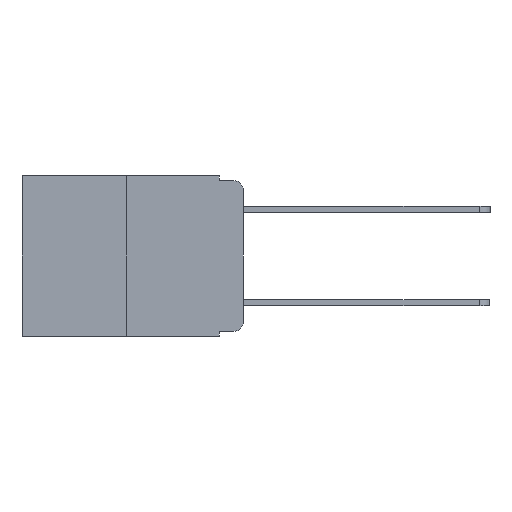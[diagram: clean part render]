
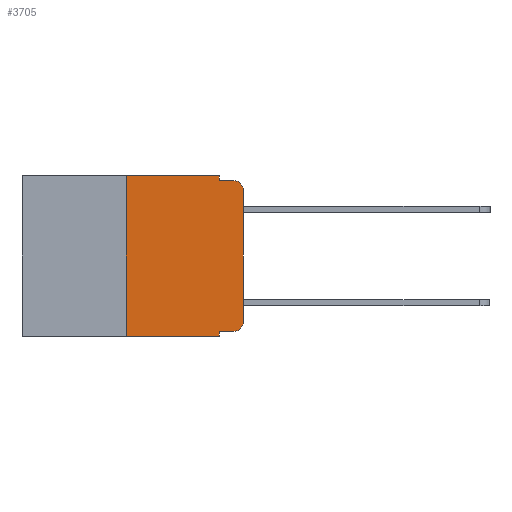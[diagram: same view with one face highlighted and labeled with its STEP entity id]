
A CAD part, left-side view. The second image highlights one B-rep face of the part: STEP entity #3705.
In plain terms, the highlighted planar face has unit normal (-1, 0, 0).
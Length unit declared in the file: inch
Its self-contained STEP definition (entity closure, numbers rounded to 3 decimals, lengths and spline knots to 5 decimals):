
#115 = DIRECTION ( 'NONE',  ( 0., 0., -1. ) ) ;
#124 = EDGE_CURVE ( 'NONE', #6362, #11952, #1915, .T. ) ;
#329 = DIRECTION ( 'NONE',  ( 0., 0., -1. ) ) ;
#531 = ORIENTED_EDGE ( 'NONE', *, *, #14129, .T. ) ;
#586 = CARTESIAN_POINT ( 'NONE',  ( 0., 0.25, -0.343 ) ) ;
#763 = ORIENTED_EDGE ( 'NONE', *, *, #14871, .F. ) ;
#785 = ORIENTED_EDGE ( 'NONE', *, *, #124, .F. ) ;
#868 = EDGE_CURVE ( 'NONE', #14524, #15082, #9923, .T. ) ;
#1090 = EDGE_CURVE ( 'NONE', #14524, #1942, #3526, .T. ) ;
#1223 = ORIENTED_EDGE ( 'NONE', *, *, #2895, .T. ) ;
#1294 = DIRECTION ( 'NONE',  ( 0., -1., 0. ) ) ;
#1351 = VECTOR ( 'NONE', #3807, 39.37008 ) ;
#1685 = DIRECTION ( 'NONE',  ( 0., 0., 1. ) ) ;
#1759 = ORIENTED_EDGE ( 'NONE', *, *, #13413, .T. ) ;
#1883 = CARTESIAN_POINT ( 'NONE',  ( 0., 0.051, 0. ) ) ;
#1915 = LINE ( 'NONE', #9579, #14061 ) ;
#1942 = VERTEX_POINT ( 'NONE', #13711 ) ;
#1986 = DIRECTION ( 'NONE',  ( 0., 0., -1. ) ) ;
#2020 = CARTESIAN_POINT ( 'NONE',  ( 0., 0.02, -0.313 ) ) ;
#2054 = EDGE_CURVE ( 'NONE', #12287, #15082, #12984, .T. ) ;
#2080 = CARTESIAN_POINT ( 'NONE',  ( 0., 0.051, -0.333 ) ) ;
#2609 = CARTESIAN_POINT ( 'NONE',  ( 0., 0.473, -0.343 ) ) ;
#2680 = VECTOR ( 'NONE', #8881, 39.37008 ) ;
#2707 = CARTESIAN_POINT ( 'NONE',  ( 0., 0.02, -0.03 ) ) ;
#2834 = CIRCLE ( 'NONE', #8735, 0.02 ) ;
#2895 = EDGE_CURVE ( 'NONE', #12287, #6593, #11436, .T. ) ;
#3144 = VECTOR ( 'NONE', #5288, 39.37008 ) ;
#3299 = DIRECTION ( 'NONE',  ( 0., 0., -1. ) ) ;
#3526 = LINE ( 'NONE', #4056, #15412 ) ;
#3614 = CARTESIAN_POINT ( 'NONE',  ( 0., 0.02, -0.333 ) ) ;
#3705 = ADVANCED_FACE ( 'NONE', ( #13661 ), #13566, .F. ) ;
#3807 = DIRECTION ( 'NONE',  ( 0., -1., 0. ) ) ;
#4014 = DIRECTION ( 'NONE',  ( 0., 0., -1. ) ) ;
#4056 = CARTESIAN_POINT ( 'NONE',  ( 0., 0.25, 0. ) ) ;
#4590 = CARTESIAN_POINT ( 'NONE',  ( 0., 0.051, 0. ) ) ;
#4902 = LINE ( 'NONE', #13055, #1351 ) ;
#5288 = DIRECTION ( 'NONE',  ( 0., -1., 0. ) ) ;
#5494 = VECTOR ( 'NONE', #1294, 39.37008 ) ;
#5897 = LINE ( 'NONE', #8769, #5494 ) ;
#5970 = AXIS2_PLACEMENT_3D ( 'NONE', #2707, #11037, #4014 ) ;
#6274 = VERTEX_POINT ( 'NONE', #7895 ) ;
#6362 = VERTEX_POINT ( 'NONE', #1883 ) ;
#6593 = VERTEX_POINT ( 'NONE', #3614 ) ;
#6866 = CARTESIAN_POINT ( 'NONE',  ( 0., 0.473, 0. ) ) ;
#7071 = CARTESIAN_POINT ( 'NONE',  ( 0., 0.051, -0.333 ) ) ;
#7285 = CARTESIAN_POINT ( 'NONE',  ( 0., 0.02, -0.01 ) ) ;
#7782 = ORIENTED_EDGE ( 'NONE', *, *, #868, .T. ) ;
#7806 = CARTESIAN_POINT ( 'NONE',  ( 0., 0.051, -0.01 ) ) ;
#7895 = CARTESIAN_POINT ( 'NONE',  ( 0., 0., -0.313 ) ) ;
#8010 = DIRECTION ( 'NONE',  ( 1., 0., 0. ) ) ;
#8550 = EDGE_LOOP ( 'NONE', ( #1759, #531, #763, #785, #9591, #9773, #7782, #13014, #1223, #10757 ) ) ;
#8564 = VERTEX_POINT ( 'NONE', #9077 ) ;
#8735 = AXIS2_PLACEMENT_3D ( 'NONE', #2020, #10465, #3299 ) ;
#8769 = CARTESIAN_POINT ( 'NONE',  ( 0., 0.473, 0. ) ) ;
#8881 = DIRECTION ( 'NONE',  ( 0., -1., 0. ) ) ;
#8891 = DIRECTION ( 'NONE',  ( 0., 0., 1. ) ) ;
#9077 = CARTESIAN_POINT ( 'NONE',  ( 0., 0., -0.03 ) ) ;
#9579 = CARTESIAN_POINT ( 'NONE',  ( 0., 0.051, 0. ) ) ;
#9591 = ORIENTED_EDGE ( 'NONE', *, *, #10877, .F. ) ;
#9773 = ORIENTED_EDGE ( 'NONE', *, *, #1090, .F. ) ;
#9851 = LINE ( 'NONE', #10196, #12804 ) ;
#9923 = LINE ( 'NONE', #2609, #3144 ) ;
#10196 = CARTESIAN_POINT ( 'NONE',  ( 0., 0., 0. ) ) ;
#10465 = DIRECTION ( 'NONE',  ( -1., 0., 0. ) ) ;
#10757 = ORIENTED_EDGE ( 'NONE', *, *, #14515, .T. ) ;
#10877 = EDGE_CURVE ( 'NONE', #1942, #6362, #5897, .T. ) ;
#11037 = DIRECTION ( 'NONE',  ( -1., 0., 0. ) ) ;
#11436 = LINE ( 'NONE', #2080, #2680 ) ;
#11498 = VERTEX_POINT ( 'NONE', #7285 ) ;
#11952 = VERTEX_POINT ( 'NONE', #7806 ) ;
#12287 = VERTEX_POINT ( 'NONE', #7071 ) ;
#12430 = CIRCLE ( 'NONE', #5970, 0.02 ) ;
#12646 = VECTOR ( 'NONE', #1986, 39.37008 ) ;
#12804 = VECTOR ( 'NONE', #1685, 39.37008 ) ;
#12984 = LINE ( 'NONE', #4590, #12646 ) ;
#13014 = ORIENTED_EDGE ( 'NONE', *, *, #2054, .F. ) ;
#13055 = CARTESIAN_POINT ( 'NONE',  ( 0., 0.051, -0.01 ) ) ;
#13413 = EDGE_CURVE ( 'NONE', #6274, #8564, #9851, .T. ) ;
#13566 = PLANE ( 'NONE',  #13887 ) ;
#13661 = FACE_OUTER_BOUND ( 'NONE', #8550, .T. ) ;
#13711 = CARTESIAN_POINT ( 'NONE',  ( 0., 0.25, 0. ) ) ;
#13887 = AXIS2_PLACEMENT_3D ( 'NONE', #6866, #8010, #329 ) ;
#14061 = VECTOR ( 'NONE', #115, 39.37008 ) ;
#14129 = EDGE_CURVE ( 'NONE', #8564, #11498, #12430, .T. ) ;
#14446 = CARTESIAN_POINT ( 'NONE',  ( 0., 0.051, -0.343 ) ) ;
#14515 = EDGE_CURVE ( 'NONE', #6593, #6274, #2834, .T. ) ;
#14524 = VERTEX_POINT ( 'NONE', #586 ) ;
#14871 = EDGE_CURVE ( 'NONE', #11952, #11498, #4902, .T. ) ;
#15082 = VERTEX_POINT ( 'NONE', #14446 ) ;
#15412 = VECTOR ( 'NONE', #8891, 39.37008 ) ;
